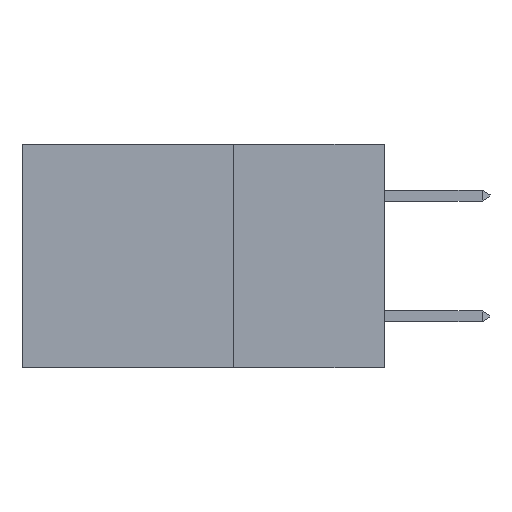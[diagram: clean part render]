
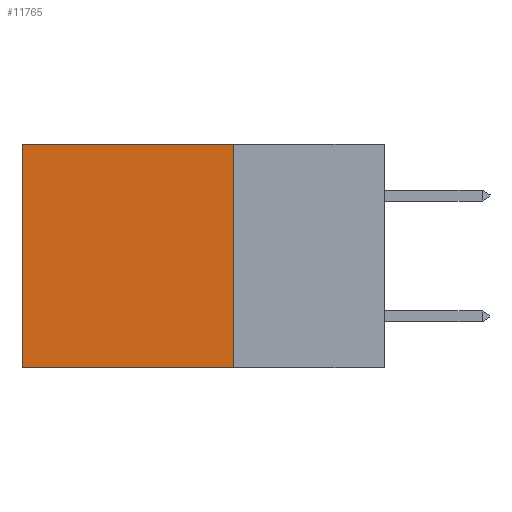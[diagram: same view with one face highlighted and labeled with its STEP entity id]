
A CAD part, left-side view. The second image highlights one B-rep face of the part: STEP entity #11765.
In plain terms, the highlighted planar face has unit normal (-1, 0, 0).
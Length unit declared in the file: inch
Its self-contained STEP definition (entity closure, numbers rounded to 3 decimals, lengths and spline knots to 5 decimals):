
#265 = ORIENTED_EDGE ( 'NONE', *, *, #4933, .F. ) ;
#837 = CARTESIAN_POINT ( 'NONE',  ( 0.2875, 0.6, 0. ) ) ;
#1358 = FACE_OUTER_BOUND ( 'NONE', #6264, .T. ) ;
#1519 = EDGE_CURVE ( 'NONE', #5959, #7081, #9514, .T. ) ;
#2213 = DIRECTION ( 'NONE',  ( 0., 1., 0. ) ) ;
#3582 = ORIENTED_EDGE ( 'NONE', *, *, #11851, .T. ) ;
#3716 = PLANE ( 'NONE',  #13833 ) ;
#3893 = CARTESIAN_POINT ( 'NONE',  ( 0.2875, 0.25, -0.37 ) ) ;
#4106 = CARTESIAN_POINT ( 'NONE',  ( 0.2875, 0.25, 0. ) ) ;
#4877 = DIRECTION ( 'NONE',  ( 0., 1., 0. ) ) ;
#4933 = EDGE_CURVE ( 'NONE', #12310, #5365, #8702, .T. ) ;
#5097 = DIRECTION ( 'NONE',  ( 0., 0., -1. ) ) ;
#5139 = DIRECTION ( 'NONE',  ( 0., 0., -1. ) ) ;
#5365 = VERTEX_POINT ( 'NONE', #10142 ) ;
#5959 = VERTEX_POINT ( 'NONE', #13187 ) ;
#6043 = DIRECTION ( 'NONE',  ( 1., 0., 0. ) ) ;
#6264 = EDGE_LOOP ( 'NONE', ( #3582, #265, #13792, #7704 ) ) ;
#6822 = VECTOR ( 'NONE', #4877, 39.37008 ) ;
#7081 = VERTEX_POINT ( 'NONE', #837 ) ;
#7096 = VECTOR ( 'NONE', #2213, 39.37008 ) ;
#7684 = LINE ( 'NONE', #4106, #8007 ) ;
#7704 = ORIENTED_EDGE ( 'NONE', *, *, #1519, .T. ) ;
#8007 = VECTOR ( 'NONE', #10689, 39.37008 ) ;
#8092 = CARTESIAN_POINT ( 'NONE',  ( 0.2875, 0.25, 0. ) ) ;
#8230 = CARTESIAN_POINT ( 'NONE',  ( 0.2875, 0.6, 0. ) ) ;
#8702 = LINE ( 'NONE', #10159, #6822 ) ;
#9514 = LINE ( 'NONE', #11112, #7096 ) ;
#9719 = LINE ( 'NONE', #8230, #10042 ) ;
#10042 = VECTOR ( 'NONE', #5097, 39.37008 ) ;
#10142 = CARTESIAN_POINT ( 'NONE',  ( 0.2875, 0.6, -0.37 ) ) ;
#10159 = CARTESIAN_POINT ( 'NONE',  ( 0.2875, 0.25, -0.37 ) ) ;
#10689 = DIRECTION ( 'NONE',  ( 0., 0., -1. ) ) ;
#11112 = CARTESIAN_POINT ( 'NONE',  ( 0.2875, 0.25, 0. ) ) ;
#11765 = ADVANCED_FACE ( 'NONE', ( #1358 ), #3716, .F. ) ;
#11851 = EDGE_CURVE ( 'NONE', #7081, #5365, #9719, .T. ) ;
#12310 = VERTEX_POINT ( 'NONE', #3893 ) ;
#13187 = CARTESIAN_POINT ( 'NONE',  ( 0.2875, 0.25, 0. ) ) ;
#13368 = EDGE_CURVE ( 'NONE', #5959, #12310, #7684, .T. ) ;
#13792 = ORIENTED_EDGE ( 'NONE', *, *, #13368, .F. ) ;
#13833 = AXIS2_PLACEMENT_3D ( 'NONE', #8092, #6043, #5139 ) ;
